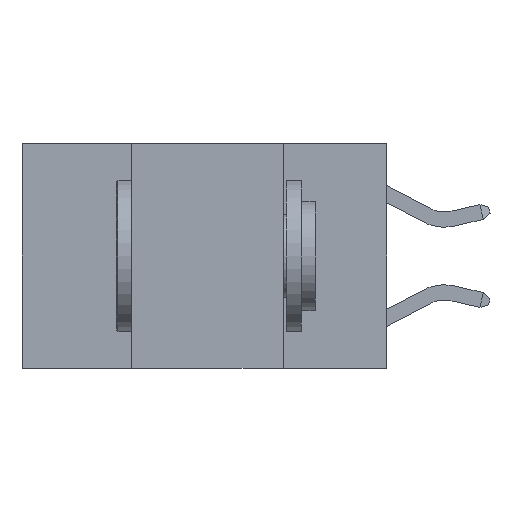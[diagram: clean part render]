
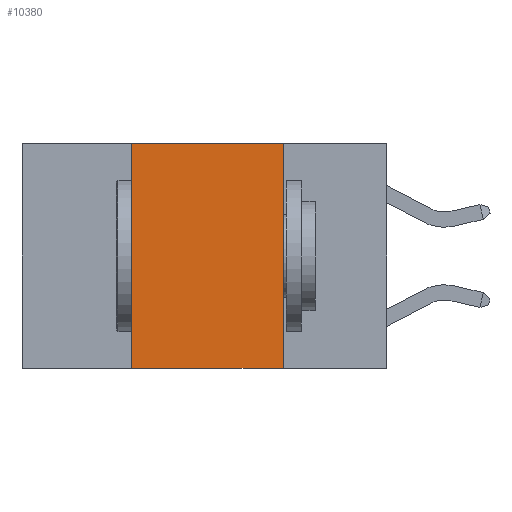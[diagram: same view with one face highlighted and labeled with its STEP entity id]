
A CAD part, left-side view. The second image highlights one B-rep face of the part: STEP entity #10380.
In plain terms, the highlighted planar face has unit normal (-1, 0, 0).
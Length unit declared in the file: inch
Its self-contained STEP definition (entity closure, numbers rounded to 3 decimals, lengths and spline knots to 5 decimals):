
#5 = CARTESIAN_POINT ( 'NONE',  ( 0., 0.17, 0. ) ) ;
#94 = DIRECTION ( 'NONE',  ( 0., 0., -1. ) ) ;
#203 = DIRECTION ( 'NONE',  ( 0., 0., -1. ) ) ;
#682 = ORIENTED_EDGE ( 'NONE', *, *, #4082, .F. ) ;
#992 = EDGE_CURVE ( 'NONE', #12922, #8889, #15217, .T. ) ;
#1229 = EDGE_LOOP ( 'NONE', ( #1637, #682, #1964, #1431 ) ) ;
#1319 = CARTESIAN_POINT ( 'NONE',  ( 0., 0.6, 0. ) ) ;
#1431 = ORIENTED_EDGE ( 'NONE', *, *, #11734, .T. ) ;
#1637 = ORIENTED_EDGE ( 'NONE', *, *, #992, .F. ) ;
#1761 = LINE ( 'NONE', #8601, #12171 ) ;
#1964 = ORIENTED_EDGE ( 'NONE', *, *, #2517, .F. ) ;
#1981 = VERTEX_POINT ( 'NONE', #9629 ) ;
#2104 = LINE ( 'NONE', #17409, #2775 ) ;
#2395 = VECTOR ( 'NONE', #94, 39.37008 ) ;
#2517 = EDGE_CURVE ( 'NONE', #8280, #1981, #1761, .T. ) ;
#2775 = VECTOR ( 'NONE', #4939, 39.37008 ) ;
#2930 = DIRECTION ( 'NONE',  ( 0., -1., 0. ) ) ;
#3401 = CARTESIAN_POINT ( 'NONE',  ( 0., 0.17, -0.37 ) ) ;
#3663 = LINE ( 'NONE', #8593, #11726 ) ;
#4082 = EDGE_CURVE ( 'NONE', #1981, #12922, #2104, .T. ) ;
#4120 = FACE_OUTER_BOUND ( 'NONE', #1229, .T. ) ;
#4939 = DIRECTION ( 'NONE',  ( 0., -1., 0. ) ) ;
#6181 = AXIS2_PLACEMENT_3D ( 'NONE', #1319, #8408, #203 ) ;
#8280 = VERTEX_POINT ( 'NONE', #11028 ) ;
#8408 = DIRECTION ( 'NONE',  ( 1., 0., 0. ) ) ;
#8593 = CARTESIAN_POINT ( 'NONE',  ( 0., 0.6, -0.37 ) ) ;
#8601 = CARTESIAN_POINT ( 'NONE',  ( 0., 0.42, 0. ) ) ;
#8889 = VERTEX_POINT ( 'NONE', #3401 ) ;
#9629 = CARTESIAN_POINT ( 'NONE',  ( 0., 0.42, 0. ) ) ;
#9687 = PLANE ( 'NONE',  #6181 ) ;
#10380 = ADVANCED_FACE ( 'NONE', ( #4120 ), #9687, .F. ) ;
#11028 = CARTESIAN_POINT ( 'NONE',  ( 0., 0.42, -0.37 ) ) ;
#11726 = VECTOR ( 'NONE', #2930, 39.37008 ) ;
#11734 = EDGE_CURVE ( 'NONE', #8280, #8889, #3663, .T. ) ;
#12171 = VECTOR ( 'NONE', #15710, 39.37008 ) ;
#12922 = VERTEX_POINT ( 'NONE', #16527 ) ;
#15217 = LINE ( 'NONE', #5, #2395 ) ;
#15710 = DIRECTION ( 'NONE',  ( 0., 0., 1. ) ) ;
#16527 = CARTESIAN_POINT ( 'NONE',  ( 0., 0.17, 0. ) ) ;
#17409 = CARTESIAN_POINT ( 'NONE',  ( 0., 0.6, 0. ) ) ;
